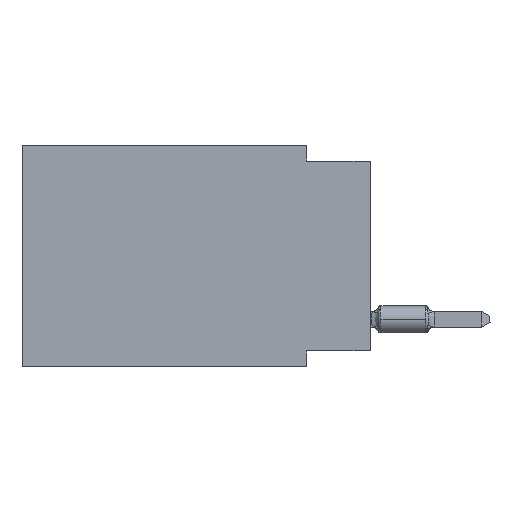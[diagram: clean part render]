
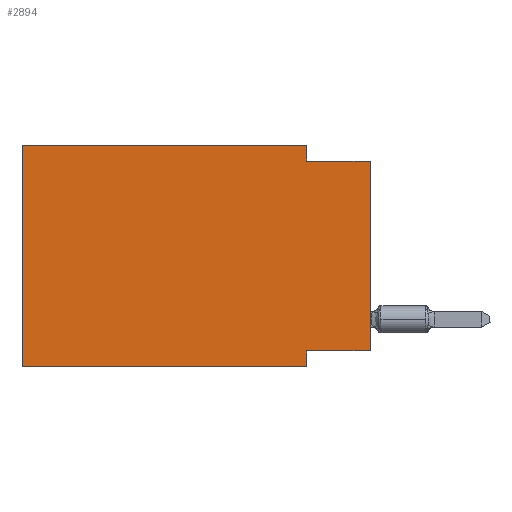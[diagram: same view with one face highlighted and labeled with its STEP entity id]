
A CAD part, left-side view. The second image highlights one B-rep face of the part: STEP entity #2894.
In plain terms, the highlighted planar face has unit normal (-1, 0, 0).
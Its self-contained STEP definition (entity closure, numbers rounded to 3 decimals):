
#25 = CARTESIAN_POINT ( 'NONE',  ( 0., 2.54, -8.255 ) ) ;
#520 = DIRECTION ( 'NONE',  ( 0., 0., -1. ) ) ;
#542 = CARTESIAN_POINT ( 'NONE',  ( 0., 0., -0.635 ) ) ;
#1102 = VECTOR ( 'NONE', #21228, 1000. ) ;
#1277 = ORIENTED_EDGE ( 'NONE', *, *, #20959, .T. ) ;
#1392 = VERTEX_POINT ( 'NONE', #25 ) ;
#1475 = ORIENTED_EDGE ( 'NONE', *, *, #25266, .F. ) ;
#1589 = ORIENTED_EDGE ( 'NONE', *, *, #14455, .F. ) ;
#1634 = CARTESIAN_POINT ( 'NONE',  ( 0., 13.97, -8.89 ) ) ;
#2894 = ADVANCED_FACE ( 'NONE', ( #6863 ), #21387, .F. ) ;
#2999 = CARTESIAN_POINT ( 'NONE',  ( 0., 13.97, 0. ) ) ;
#3105 = LINE ( 'NONE', #15971, #16893 ) ;
#3302 = EDGE_CURVE ( 'NONE', #20134, #4034, #21488, .T. ) ;
#4034 = VERTEX_POINT ( 'NONE', #542 ) ;
#4964 = EDGE_CURVE ( 'NONE', #20134, #1392, #3105, .T. ) ;
#5709 = DIRECTION ( 'NONE',  ( 0., 1., 0. ) ) ;
#6189 = EDGE_CURVE ( 'NONE', #1392, #9999, #21123, .T. ) ;
#6781 = CARTESIAN_POINT ( 'NONE',  ( 0., 2.54, 0. ) ) ;
#6863 = FACE_OUTER_BOUND ( 'NONE', #7180, .T. ) ;
#7180 = EDGE_LOOP ( 'NONE', ( #7337, #1475, #13874, #17960, #1589, #1277, #12463, #14713 ) ) ;
#7182 = DIRECTION ( 'NONE',  ( 0., -1., 0. ) ) ;
#7337 = ORIENTED_EDGE ( 'NONE', *, *, #3302, .T. ) ;
#8368 = LINE ( 'NONE', #10727, #19639 ) ;
#9361 = DIRECTION ( 'NONE',  ( 0., 0., -1. ) ) ;
#9451 = CARTESIAN_POINT ( 'NONE',  ( 0., 2.54, -0.635 ) ) ;
#9832 = VECTOR ( 'NONE', #27198, 1000. ) ;
#9999 = VERTEX_POINT ( 'NONE', #26987 ) ;
#10076 = CARTESIAN_POINT ( 'NONE',  ( 0., 13.97, -8.89 ) ) ;
#10201 = LINE ( 'NONE', #1634, #9832 ) ;
#10631 = VECTOR ( 'NONE', #25923, 1000. ) ;
#10727 = CARTESIAN_POINT ( 'NONE',  ( 0., 13.97, 0. ) ) ;
#10889 = DIRECTION ( 'NONE',  ( 1., 0., 0. ) ) ;
#11155 = DIRECTION ( 'NONE',  ( 0., 0., 1. ) ) ;
#11305 = LINE ( 'NONE', #2999, #13993 ) ;
#12463 = ORIENTED_EDGE ( 'NONE', *, *, #6189, .F. ) ;
#12678 = EDGE_CURVE ( 'NONE', #20791, #21561, #8368, .T. ) ;
#13430 = LINE ( 'NONE', #16040, #16061 ) ;
#13874 = ORIENTED_EDGE ( 'NONE', *, *, #25899, .F. ) ;
#13993 = VECTOR ( 'NONE', #11155, 1000. ) ;
#14455 = EDGE_CURVE ( 'NONE', #19823, #20791, #11305, .T. ) ;
#14713 = ORIENTED_EDGE ( 'NONE', *, *, #4964, .F. ) ;
#15971 = CARTESIAN_POINT ( 'NONE',  ( 0., 0., -8.255 ) ) ;
#16040 = CARTESIAN_POINT ( 'NONE',  ( 0., 0., -0.635 ) ) ;
#16061 = VECTOR ( 'NONE', #7182, 1000. ) ;
#16674 = VERTEX_POINT ( 'NONE', #9451 ) ;
#16778 = CARTESIAN_POINT ( 'NONE',  ( 0., 0., -8.255 ) ) ;
#16893 = VECTOR ( 'NONE', #5709, 1000. ) ;
#17247 = CARTESIAN_POINT ( 'NONE',  ( 0., 13.97, 0. ) ) ;
#17960 = ORIENTED_EDGE ( 'NONE', *, *, #12678, .F. ) ;
#19124 = VECTOR ( 'NONE', #520, 1000. ) ;
#19154 = DIRECTION ( 'NONE',  ( 0., -1., 0. ) ) ;
#19418 = CARTESIAN_POINT ( 'NONE',  ( 0., 0., 0. ) ) ;
#19639 = VECTOR ( 'NONE', #19154, 1000. ) ;
#19823 = VERTEX_POINT ( 'NONE', #10076 ) ;
#20134 = VERTEX_POINT ( 'NONE', #16778 ) ;
#20791 = VERTEX_POINT ( 'NONE', #26534 ) ;
#20959 = EDGE_CURVE ( 'NONE', #19823, #9999, #10201, .T. ) ;
#21123 = LINE ( 'NONE', #25409, #19124 ) ;
#21228 = DIRECTION ( 'NONE',  ( 0., 0., -1. ) ) ;
#21387 = PLANE ( 'NONE',  #24741 ) ;
#21488 = LINE ( 'NONE', #19418, #10631 ) ;
#21561 = VERTEX_POINT ( 'NONE', #6781 ) ;
#24741 = AXIS2_PLACEMENT_3D ( 'NONE', #17247, #10889, #9361 ) ;
#25266 = EDGE_CURVE ( 'NONE', #16674, #4034, #13430, .T. ) ;
#25409 = CARTESIAN_POINT ( 'NONE',  ( 0., 2.54, -8.89 ) ) ;
#25514 = LINE ( 'NONE', #27327, #1102 ) ;
#25899 = EDGE_CURVE ( 'NONE', #21561, #16674, #25514, .T. ) ;
#25923 = DIRECTION ( 'NONE',  ( 0., 0., 1. ) ) ;
#26534 = CARTESIAN_POINT ( 'NONE',  ( 0., 13.97, 0. ) ) ;
#26987 = CARTESIAN_POINT ( 'NONE',  ( 0., 2.54, -8.89 ) ) ;
#27198 = DIRECTION ( 'NONE',  ( 0., -1., 0. ) ) ;
#27327 = CARTESIAN_POINT ( 'NONE',  ( 0., 2.54, 0. ) ) ;
